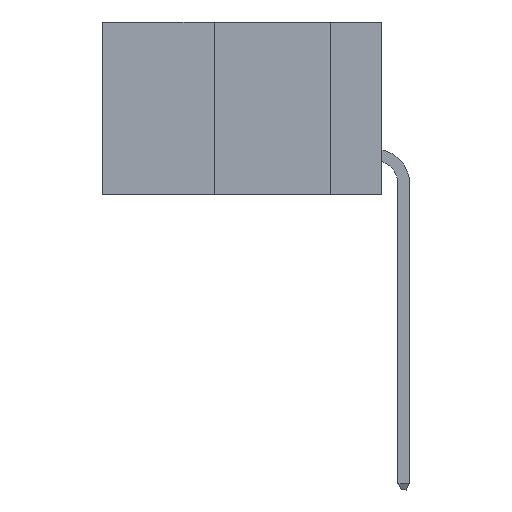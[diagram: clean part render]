
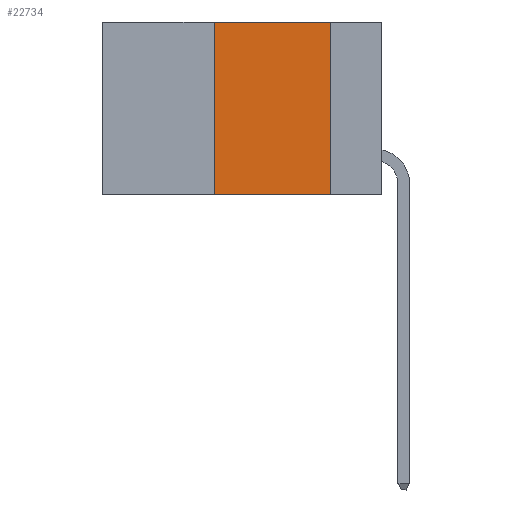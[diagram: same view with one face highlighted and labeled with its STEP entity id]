
A CAD part, left-side view. The second image highlights one B-rep face of the part: STEP entity #22734.
In plain terms, the highlighted planar face has unit normal (-1, 0, 0).
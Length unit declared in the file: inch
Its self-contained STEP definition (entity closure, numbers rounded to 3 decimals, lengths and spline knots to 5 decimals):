
#1519 = CARTESIAN_POINT ( 'NONE',  ( 0., 0.6, -0.37 ) ) ;
#9675 = DIRECTION ( 'NONE',  ( 0., 0., -1. ) ) ;
#9879 = LINE ( 'NONE', #30620, #31535 ) ;
#10221 = EDGE_CURVE ( 'NONE', #18707, #34238, #27859, .T. ) ;
#12851 = EDGE_CURVE ( 'NONE', #22410, #34238, #37090, .T. ) ;
#14810 = AXIS2_PLACEMENT_3D ( 'NONE', #20279, #37041, #21822 ) ;
#14960 = ORIENTED_EDGE ( 'NONE', *, *, #12851, .T. ) ;
#15181 = CARTESIAN_POINT ( 'NONE',  ( 0., 0.36, -0.37 ) ) ;
#15464 = DIRECTION ( 'NONE',  ( 0., -1., 0. ) ) ;
#15940 = DIRECTION ( 'NONE',  ( 0., -1., 0. ) ) ;
#17786 = CARTESIAN_POINT ( 'NONE',  ( 0., 0.36, 0. ) ) ;
#18049 = ORIENTED_EDGE ( 'NONE', *, *, #10221, .F. ) ;
#18555 = CARTESIAN_POINT ( 'NONE',  ( 0., 0.11, 0. ) ) ;
#18707 = VERTEX_POINT ( 'NONE', #22536 ) ;
#20279 = CARTESIAN_POINT ( 'NONE',  ( 0., 0.6, 0. ) ) ;
#20807 = ORIENTED_EDGE ( 'NONE', *, *, #28577, .F. ) ;
#21011 = LINE ( 'NONE', #21583, #27175 ) ;
#21583 = CARTESIAN_POINT ( 'NONE',  ( 0., 0.6, 0. ) ) ;
#21822 = DIRECTION ( 'NONE',  ( 0., 0., -1. ) ) ;
#22410 = VERTEX_POINT ( 'NONE', #15181 ) ;
#22536 = CARTESIAN_POINT ( 'NONE',  ( 0., 0.11, 0. ) ) ;
#22734 = ADVANCED_FACE ( 'NONE', ( #38069 ), #32134, .F. ) ;
#24087 = EDGE_LOOP ( 'NONE', ( #18049, #28121, #20807, #14960 ) ) ;
#24451 = VECTOR ( 'NONE', #15940, 39.37008 ) ;
#26160 = VERTEX_POINT ( 'NONE', #17786 ) ;
#27175 = VECTOR ( 'NONE', #15464, 39.37008 ) ;
#27859 = LINE ( 'NONE', #18555, #35912 ) ;
#28121 = ORIENTED_EDGE ( 'NONE', *, *, #29867, .F. ) ;
#28577 = EDGE_CURVE ( 'NONE', #22410, #26160, #9879, .T. ) ;
#29867 = EDGE_CURVE ( 'NONE', #26160, #18707, #21011, .T. ) ;
#30620 = CARTESIAN_POINT ( 'NONE',  ( 0., 0.36, 0. ) ) ;
#31269 = CARTESIAN_POINT ( 'NONE',  ( 0., 0.11, -0.37 ) ) ;
#31535 = VECTOR ( 'NONE', #33792, 39.37008 ) ;
#32134 = PLANE ( 'NONE',  #14810 ) ;
#33792 = DIRECTION ( 'NONE',  ( 0., 0., 1. ) ) ;
#34238 = VERTEX_POINT ( 'NONE', #31269 ) ;
#35912 = VECTOR ( 'NONE', #9675, 39.37008 ) ;
#37041 = DIRECTION ( 'NONE',  ( 1., 0., 0. ) ) ;
#37090 = LINE ( 'NONE', #1519, #24451 ) ;
#38069 = FACE_OUTER_BOUND ( 'NONE', #24087, .T. ) ;
